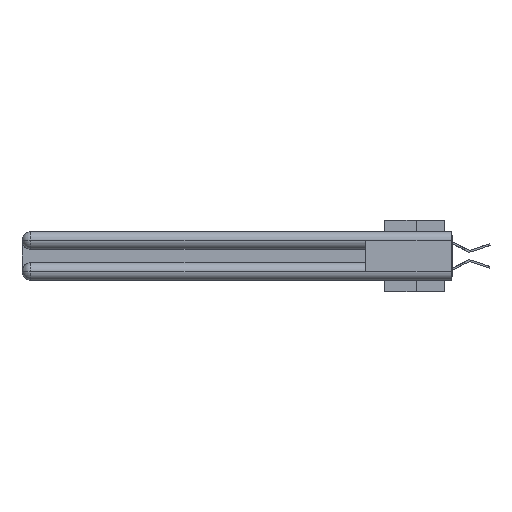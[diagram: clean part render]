
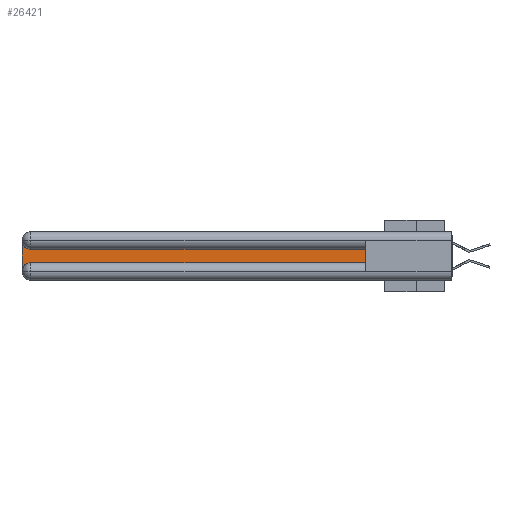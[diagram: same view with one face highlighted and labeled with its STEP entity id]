
A CAD part, left-side view. The second image highlights one B-rep face of the part: STEP entity #26421.
In plain terms, the highlighted planar face has unit normal (-1, 0, 0).
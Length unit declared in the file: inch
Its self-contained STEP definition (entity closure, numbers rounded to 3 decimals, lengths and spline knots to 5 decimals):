
#138 = DIRECTION ( 'NONE',  ( 0., 0., -1. ) ) ;
#1968 = VERTEX_POINT ( 'NONE', #26702 ) ;
#2101 = CARTESIAN_POINT ( 'NONE',  ( 0.075, 0.6, -0.2175 ) ) ;
#2456 = EDGE_LOOP ( 'NONE', ( #37014, #17033, #32191, #20647, #5097, #8437 ) ) ;
#3382 = VERTEX_POINT ( 'NONE', #30913 ) ;
#3567 = DIRECTION ( 'NONE',  ( 1., 0., 0. ) ) ;
#3964 = EDGE_CURVE ( 'NONE', #3382, #34367, #34974, .T. ) ;
#4239 = EDGE_CURVE ( 'NONE', #34367, #33005, #38737, .T. ) ;
#4716 = DIRECTION ( 'NONE',  ( 0., -1., 0. ) ) ;
#5097 = ORIENTED_EDGE ( 'NONE', *, *, #4239, .T. ) ;
#7526 = EDGE_CURVE ( 'NONE', #33005, #1968, #17968, .T. ) ;
#8437 = ORIENTED_EDGE ( 'NONE', *, *, #7526, .T. ) ;
#9707 = DIRECTION ( 'NONE',  ( 0., 1., 0. ) ) ;
#13377 = DIRECTION ( 'NONE',  ( 0., 0., -1. ) ) ;
#13577 = AXIS2_PLACEMENT_3D ( 'NONE', #36581, #3567, #138 ) ;
#14021 = EDGE_CURVE ( 'NONE', #19031, #3382, #33589, .T. ) ;
#15530 = DIRECTION ( 'NONE',  ( 0., 0., 1. ) ) ;
#15630 = EDGE_CURVE ( 'NONE', #35931, #19031, #27670, .T. ) ;
#16188 = DIRECTION ( 'NONE',  ( 1., 0., 0. ) ) ;
#17033 = ORIENTED_EDGE ( 'NONE', *, *, #15630, .T. ) ;
#17219 = CARTESIAN_POINT ( 'NONE',  ( 0.075, 3., -0.0625 ) ) ;
#17659 = AXIS2_PLACEMENT_3D ( 'NONE', #22405, #16188, #13377 ) ;
#17968 = LINE ( 'NONE', #33627, #18938 ) ;
#18319 = CARTESIAN_POINT ( 'NONE',  ( 0.075, 3., -0.2175 ) ) ;
#18673 = FACE_OUTER_BOUND ( 'NONE', #2456, .T. ) ;
#18938 = VECTOR ( 'NONE', #15530, 39.37008 ) ;
#19031 = VERTEX_POINT ( 'NONE', #17219 ) ;
#19360 = CARTESIAN_POINT ( 'NONE',  ( 0.075, 0.6, -0.1225 ) ) ;
#20647 = ORIENTED_EDGE ( 'NONE', *, *, #3964, .T. ) ;
#21479 = CARTESIAN_POINT ( 'NONE',  ( 0.075, 3., -0.1225 ) ) ;
#22405 = CARTESIAN_POINT ( 'NONE',  ( 0.075, 2.94, -0.2775 ) ) ;
#26421 = ADVANCED_FACE ( 'NONE', ( #18673 ), #30935, .F. ) ;
#26575 = CARTESIAN_POINT ( 'NONE',  ( 0.075, 2.94, -0.1225 ) ) ;
#26702 = CARTESIAN_POINT ( 'NONE',  ( 0.075, 0.6, -0.1225 ) ) ;
#27670 = CIRCLE ( 'NONE', #13577, 0.06 ) ;
#30072 = AXIS2_PLACEMENT_3D ( 'NONE', #21479, #39619, #33949 ) ;
#30190 = VECTOR ( 'NONE', #39658, 39.37008 ) ;
#30553 = EDGE_CURVE ( 'NONE', #1968, #35931, #34846, .T. ) ;
#30880 = VECTOR ( 'NONE', #9707, 39.37008 ) ;
#30913 = CARTESIAN_POINT ( 'NONE',  ( 0.075, 3., -0.2775 ) ) ;
#30935 = PLANE ( 'NONE',  #30072 ) ;
#32191 = ORIENTED_EDGE ( 'NONE', *, *, #14021, .T. ) ;
#32469 = CARTESIAN_POINT ( 'NONE',  ( 0.075, 2.94, -0.2175 ) ) ;
#32701 = CARTESIAN_POINT ( 'NONE',  ( 0.075, 0.6, -0.2175 ) ) ;
#33005 = VERTEX_POINT ( 'NONE', #32701 ) ;
#33589 = LINE ( 'NONE', #18319, #30190 ) ;
#33627 = CARTESIAN_POINT ( 'NONE',  ( 0.075, 0.6, -0.2175 ) ) ;
#33949 = DIRECTION ( 'NONE',  ( 0., 0., -1. ) ) ;
#34367 = VERTEX_POINT ( 'NONE', #32469 ) ;
#34846 = LINE ( 'NONE', #19360, #30880 ) ;
#34974 = CIRCLE ( 'NONE', #17659, 0.06 ) ;
#35931 = VERTEX_POINT ( 'NONE', #26575 ) ;
#36581 = CARTESIAN_POINT ( 'NONE',  ( 0.075, 2.94, -0.0625 ) ) ;
#37014 = ORIENTED_EDGE ( 'NONE', *, *, #30553, .T. ) ;
#37571 = VECTOR ( 'NONE', #4716, 39.37008 ) ;
#38737 = LINE ( 'NONE', #2101, #37571 ) ;
#39619 = DIRECTION ( 'NONE',  ( 1., 0., 0. ) ) ;
#39658 = DIRECTION ( 'NONE',  ( 0., 0., -1. ) ) ;
